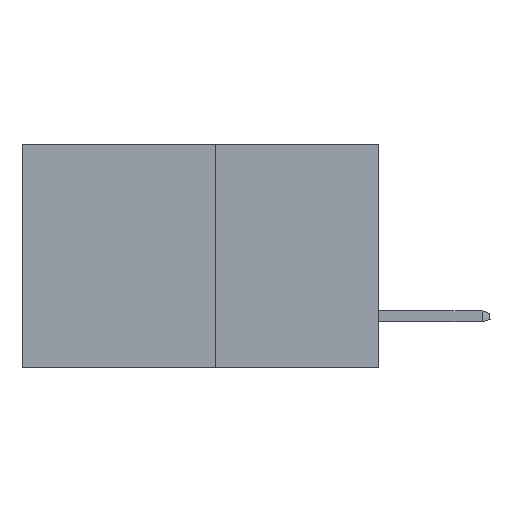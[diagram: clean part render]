
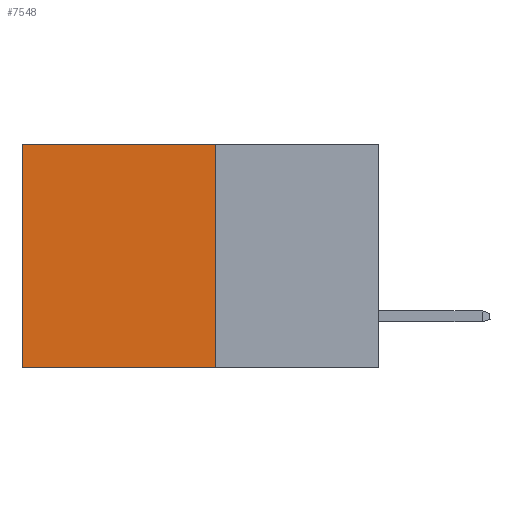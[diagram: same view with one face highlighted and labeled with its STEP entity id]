
A CAD part, left-side view. The second image highlights one B-rep face of the part: STEP entity #7548.
In plain terms, the highlighted planar face has unit normal (-1, 0, 0).
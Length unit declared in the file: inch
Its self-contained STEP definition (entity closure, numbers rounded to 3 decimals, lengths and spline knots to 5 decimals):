
#38 = CARTESIAN_POINT ( 'NONE',  ( 0.277, 0.27, -0.37 ) ) ;
#126 = DIRECTION ( 'NONE',  ( 0., 0., -1. ) ) ;
#1336 = VERTEX_POINT ( 'NONE', #7794 ) ;
#2069 = EDGE_CURVE ( 'NONE', #9093, #13348, #13745, .T. ) ;
#2359 = DIRECTION ( 'NONE',  ( 0., 1., 0. ) ) ;
#2394 = EDGE_CURVE ( 'NONE', #13348, #1336, #14701, .T. ) ;
#3425 = VECTOR ( 'NONE', #2359, 39.37008 ) ;
#3457 = DIRECTION ( 'NONE',  ( 0., 0., -1. ) ) ;
#3762 = DIRECTION ( 'NONE',  ( 1., 0., 0. ) ) ;
#4985 = CARTESIAN_POINT ( 'NONE',  ( 0.277, 0.27, -0.37 ) ) ;
#5275 = ORIENTED_EDGE ( 'NONE', *, *, #8190, .F. ) ;
#5595 = VERTEX_POINT ( 'NONE', #38 ) ;
#7047 = VECTOR ( 'NONE', #126, 39.37008 ) ;
#7548 = ADVANCED_FACE ( 'NONE', ( #10219 ), #12818, .F. ) ;
#7794 = CARTESIAN_POINT ( 'NONE',  ( 0.277, 0.59, -0.37 ) ) ;
#8190 = EDGE_CURVE ( 'NONE', #5595, #1336, #9506, .T. ) ;
#8358 = CARTESIAN_POINT ( 'NONE',  ( 0.277, 0.27, -0.37 ) ) ;
#8405 = EDGE_CURVE ( 'NONE', #9093, #5595, #10025, .T. ) ;
#8539 = ORIENTED_EDGE ( 'NONE', *, *, #2069, .T. ) ;
#9093 = VERTEX_POINT ( 'NONE', #13012 ) ;
#9281 = CARTESIAN_POINT ( 'NONE',  ( 0.277, 0.27, -0.37 ) ) ;
#9506 = LINE ( 'NONE', #9281, #3425 ) ;
#10025 = LINE ( 'NONE', #4985, #7047 ) ;
#10219 = FACE_OUTER_BOUND ( 'NONE', #12363, .T. ) ;
#11125 = VECTOR ( 'NONE', #13437, 39.37008 ) ;
#11734 = DIRECTION ( 'NONE',  ( 0., 0., -1. ) ) ;
#11756 = VECTOR ( 'NONE', #3457, 39.37008 ) ;
#11764 = AXIS2_PLACEMENT_3D ( 'NONE', #8358, #3762, #11734 ) ;
#12134 = CARTESIAN_POINT ( 'NONE',  ( 0.277, 0.59, 0. ) ) ;
#12363 = EDGE_LOOP ( 'NONE', ( #14820, #5275, #13568, #8539 ) ) ;
#12818 = PLANE ( 'NONE',  #11764 ) ;
#13012 = CARTESIAN_POINT ( 'NONE',  ( 0.277, 0.27, 0. ) ) ;
#13050 = CARTESIAN_POINT ( 'NONE',  ( 0.277, 0.27, 0. ) ) ;
#13151 = CARTESIAN_POINT ( 'NONE',  ( 0.277, 0.59, -0.37 ) ) ;
#13348 = VERTEX_POINT ( 'NONE', #12134 ) ;
#13437 = DIRECTION ( 'NONE',  ( 0., 1., 0. ) ) ;
#13568 = ORIENTED_EDGE ( 'NONE', *, *, #8405, .F. ) ;
#13745 = LINE ( 'NONE', #13050, #11125 ) ;
#14701 = LINE ( 'NONE', #13151, #11756 ) ;
#14820 = ORIENTED_EDGE ( 'NONE', *, *, #2394, .T. ) ;
